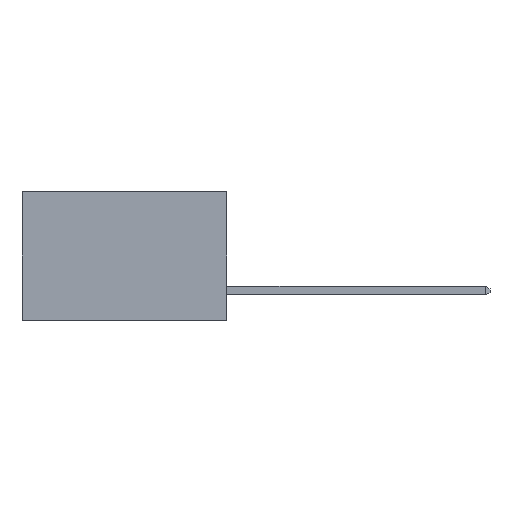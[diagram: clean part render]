
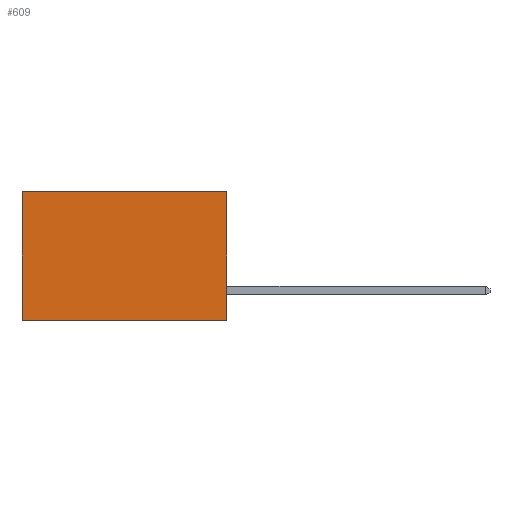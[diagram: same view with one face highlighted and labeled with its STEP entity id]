
A CAD part, left-side view. The second image highlights one B-rep face of the part: STEP entity #609.
In plain terms, the highlighted planar face has unit normal (-1, 0, 0).
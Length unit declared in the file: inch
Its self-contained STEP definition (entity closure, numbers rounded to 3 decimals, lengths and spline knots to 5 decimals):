
#299 = CARTESIAN_POINT ( 'NONE',  ( 0.277, 0., -0.37 ) ) ;
#609 = ADVANCED_FACE ( 'NONE', ( #3969 ), #6656, .F. ) ;
#962 = DIRECTION ( 'NONE',  ( 0., 0., -1. ) ) ;
#1153 = EDGE_LOOP ( 'NONE', ( #8509, #5876, #6933, #1519 ) ) ;
#1400 = EDGE_CURVE ( 'NONE', #6087, #3231, #6291, .T. ) ;
#1466 = LINE ( 'NONE', #3841, #4892 ) ;
#1519 = ORIENTED_EDGE ( 'NONE', *, *, #8105, .T. ) ;
#1911 = CARTESIAN_POINT ( 'NONE',  ( 0.277, 0., 0. ) ) ;
#2641 = CARTESIAN_POINT ( 'NONE',  ( 0.277, 0.59, -0.37 ) ) ;
#2808 = VERTEX_POINT ( 'NONE', #2641 ) ;
#2990 = VERTEX_POINT ( 'NONE', #3755 ) ;
#3231 = VERTEX_POINT ( 'NONE', #299 ) ;
#3247 = CARTESIAN_POINT ( 'NONE',  ( 0.277, 0., -0.37 ) ) ;
#3334 = CARTESIAN_POINT ( 'NONE',  ( 0.277, 0., -0.37 ) ) ;
#3755 = CARTESIAN_POINT ( 'NONE',  ( 0.277, 0.59, 0. ) ) ;
#3841 = CARTESIAN_POINT ( 'NONE',  ( 0.277, 0.59, -0.37 ) ) ;
#3900 = EDGE_CURVE ( 'NONE', #3231, #2808, #7667, .T. ) ;
#3969 = FACE_OUTER_BOUND ( 'NONE', #1153, .T. ) ;
#4237 = DIRECTION ( 'NONE',  ( 0., 1., 0. ) ) ;
#4552 = DIRECTION ( 'NONE',  ( 0., 0., -1. ) ) ;
#4892 = VECTOR ( 'NONE', #4552, 39.37008 ) ;
#5161 = AXIS2_PLACEMENT_3D ( 'NONE', #6328, #6916, #962 ) ;
#5353 = CARTESIAN_POINT ( 'NONE',  ( 0.277, 0., 0. ) ) ;
#5876 = ORIENTED_EDGE ( 'NONE', *, *, #3900, .F. ) ;
#6018 = DIRECTION ( 'NONE',  ( 0., 1., 0. ) ) ;
#6087 = VERTEX_POINT ( 'NONE', #1911 ) ;
#6291 = LINE ( 'NONE', #3334, #6508 ) ;
#6328 = CARTESIAN_POINT ( 'NONE',  ( 0.277, 0., -0.37 ) ) ;
#6508 = VECTOR ( 'NONE', #9151, 39.37008 ) ;
#6656 = PLANE ( 'NONE',  #5161 ) ;
#6916 = DIRECTION ( 'NONE',  ( 1., 0., 0. ) ) ;
#6933 = ORIENTED_EDGE ( 'NONE', *, *, #1400, .F. ) ;
#7667 = LINE ( 'NONE', #3247, #9031 ) ;
#7903 = EDGE_CURVE ( 'NONE', #2990, #2808, #1466, .T. ) ;
#8105 = EDGE_CURVE ( 'NONE', #6087, #2990, #8473, .T. ) ;
#8473 = LINE ( 'NONE', #5353, #8909 ) ;
#8509 = ORIENTED_EDGE ( 'NONE', *, *, #7903, .T. ) ;
#8909 = VECTOR ( 'NONE', #6018, 39.37008 ) ;
#9031 = VECTOR ( 'NONE', #4237, 39.37008 ) ;
#9151 = DIRECTION ( 'NONE',  ( 0., 0., -1. ) ) ;
